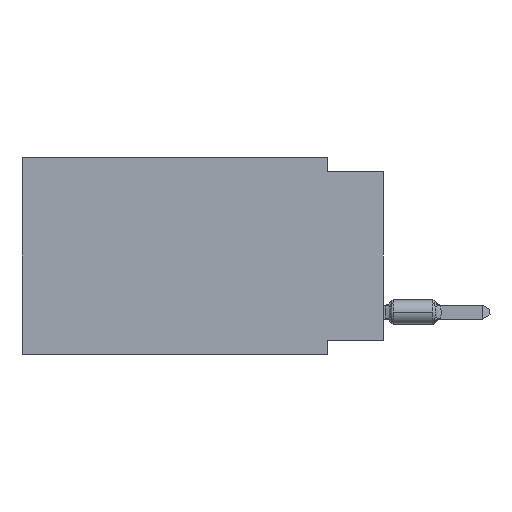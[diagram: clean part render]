
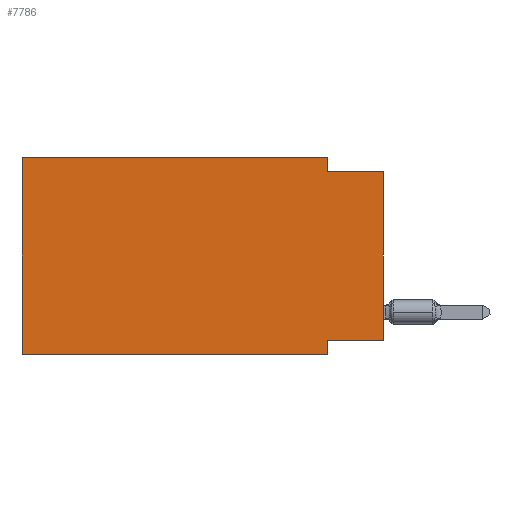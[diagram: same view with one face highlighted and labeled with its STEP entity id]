
A CAD part, left-side view. The second image highlights one B-rep face of the part: STEP entity #7786.
In plain terms, the highlighted planar face has unit normal (-1, 0, 0).
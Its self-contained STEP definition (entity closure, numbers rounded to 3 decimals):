
#46 = VERTEX_POINT ( 'NONE', #6389 ) ;
#342 = CARTESIAN_POINT ( 'NONE',  ( 0., 2.54, -8.89 ) ) ;
#832 = VERTEX_POINT ( 'NONE', #2004 ) ;
#1599 = ORIENTED_EDGE ( 'NONE', *, *, #12277, .T. ) ;
#1944 = EDGE_CURVE ( 'NONE', #3278, #13483, #8148, .T. ) ;
#2004 = CARTESIAN_POINT ( 'NONE',  ( 0., 16.383, -8.89 ) ) ;
#2079 = VECTOR ( 'NONE', #14512, 1000. ) ;
#2639 = EDGE_CURVE ( 'NONE', #46, #5056, #5601, .T. ) ;
#2804 = DIRECTION ( 'NONE',  ( 0., -1., 0. ) ) ;
#2808 = VERTEX_POINT ( 'NONE', #8416 ) ;
#3278 = VERTEX_POINT ( 'NONE', #12356 ) ;
#3581 = DIRECTION ( 'NONE',  ( 0., 0., 1. ) ) ;
#3723 = DIRECTION ( 'NONE',  ( 0., 0., -1. ) ) ;
#3873 = CARTESIAN_POINT ( 'NONE',  ( 0., 2.54, 0. ) ) ;
#4033 = VECTOR ( 'NONE', #11958, 1000. ) ;
#4061 = VECTOR ( 'NONE', #3723, 1000. ) ;
#4671 = CARTESIAN_POINT ( 'NONE',  ( 0., 0., -8.255 ) ) ;
#4775 = ORIENTED_EDGE ( 'NONE', *, *, #11190, .F. ) ;
#4830 = LINE ( 'NONE', #8467, #13561 ) ;
#5056 = VERTEX_POINT ( 'NONE', #13047 ) ;
#5196 = ORIENTED_EDGE ( 'NONE', *, *, #8891, .F. ) ;
#5601 = LINE ( 'NONE', #12873, #11112 ) ;
#5634 = ORIENTED_EDGE ( 'NONE', *, *, #14992, .F. ) ;
#5701 = EDGE_CURVE ( 'NONE', #832, #10786, #10336, .T. ) ;
#6389 = CARTESIAN_POINT ( 'NONE',  ( 0., 2.54, -0.635 ) ) ;
#6448 = LINE ( 'NONE', #3873, #4061 ) ;
#7364 = VECTOR ( 'NONE', #12034, 1000. ) ;
#7786 = ADVANCED_FACE ( 'NONE', ( #16006 ), #15004, .F. ) ;
#8148 = LINE ( 'NONE', #4671, #7364 ) ;
#8255 = VECTOR ( 'NONE', #2804, 1000. ) ;
#8402 = CARTESIAN_POINT ( 'NONE',  ( 0., 16.383, 0. ) ) ;
#8416 = CARTESIAN_POINT ( 'NONE',  ( 0., 16.383, 0. ) ) ;
#8467 = CARTESIAN_POINT ( 'NONE',  ( 0., 0., 0. ) ) ;
#8858 = ORIENTED_EDGE ( 'NONE', *, *, #2639, .F. ) ;
#8891 = EDGE_CURVE ( 'NONE', #13483, #10786, #10645, .T. ) ;
#9172 = CARTESIAN_POINT ( 'NONE',  ( 0., 16.383, -8.89 ) ) ;
#9309 = CARTESIAN_POINT ( 'NONE',  ( 0., 2.54, -8.89 ) ) ;
#9325 = VERTEX_POINT ( 'NONE', #10457 ) ;
#9472 = LINE ( 'NONE', #10961, #2079 ) ;
#9732 = CARTESIAN_POINT ( 'NONE',  ( 0., 16.383, 0. ) ) ;
#10336 = LINE ( 'NONE', #9172, #8255 ) ;
#10457 = CARTESIAN_POINT ( 'NONE',  ( 0., 2.54, 0. ) ) ;
#10645 = LINE ( 'NONE', #9309, #4033 ) ;
#10729 = CARTESIAN_POINT ( 'NONE',  ( 0., 2.54, -8.255 ) ) ;
#10786 = VERTEX_POINT ( 'NONE', #342 ) ;
#10961 = CARTESIAN_POINT ( 'NONE',  ( 0., 16.383, 0. ) ) ;
#10982 = LINE ( 'NONE', #9732, #16331 ) ;
#11112 = VECTOR ( 'NONE', #15354, 1000. ) ;
#11190 = EDGE_CURVE ( 'NONE', #9325, #46, #6448, .T. ) ;
#11576 = ORIENTED_EDGE ( 'NONE', *, *, #5701, .T. ) ;
#11958 = DIRECTION ( 'NONE',  ( 0., 0., -1. ) ) ;
#12034 = DIRECTION ( 'NONE',  ( 0., 1., 0. ) ) ;
#12123 = DIRECTION ( 'NONE',  ( 1., 0., 0. ) ) ;
#12277 = EDGE_CURVE ( 'NONE', #3278, #5056, #4830, .T. ) ;
#12356 = CARTESIAN_POINT ( 'NONE',  ( 0., 0., -8.255 ) ) ;
#12873 = CARTESIAN_POINT ( 'NONE',  ( 0., 0., -0.635 ) ) ;
#13047 = CARTESIAN_POINT ( 'NONE',  ( 0., 0., -0.635 ) ) ;
#13483 = VERTEX_POINT ( 'NONE', #10729 ) ;
#13561 = VECTOR ( 'NONE', #3581, 1000. ) ;
#14038 = AXIS2_PLACEMENT_3D ( 'NONE', #8402, #12123, #14686 ) ;
#14227 = ORIENTED_EDGE ( 'NONE', *, *, #14628, .F. ) ;
#14512 = DIRECTION ( 'NONE',  ( 0., -1., 0. ) ) ;
#14627 = ORIENTED_EDGE ( 'NONE', *, *, #1944, .F. ) ;
#14628 = EDGE_CURVE ( 'NONE', #832, #2808, #10982, .T. ) ;
#14686 = DIRECTION ( 'NONE',  ( 0., 0., -1. ) ) ;
#14777 = DIRECTION ( 'NONE',  ( 0., 0., 1. ) ) ;
#14992 = EDGE_CURVE ( 'NONE', #2808, #9325, #9472, .T. ) ;
#15004 = PLANE ( 'NONE',  #14038 ) ;
#15049 = EDGE_LOOP ( 'NONE', ( #1599, #8858, #4775, #5634, #14227, #11576, #5196, #14627 ) ) ;
#15354 = DIRECTION ( 'NONE',  ( 0., -1., 0. ) ) ;
#16006 = FACE_OUTER_BOUND ( 'NONE', #15049, .T. ) ;
#16331 = VECTOR ( 'NONE', #14777, 1000. ) ;
